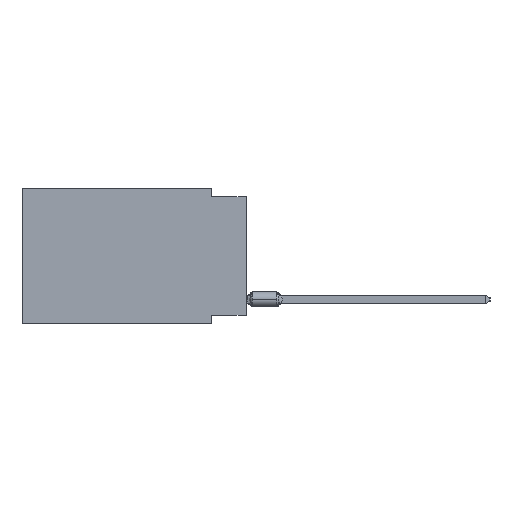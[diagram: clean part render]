
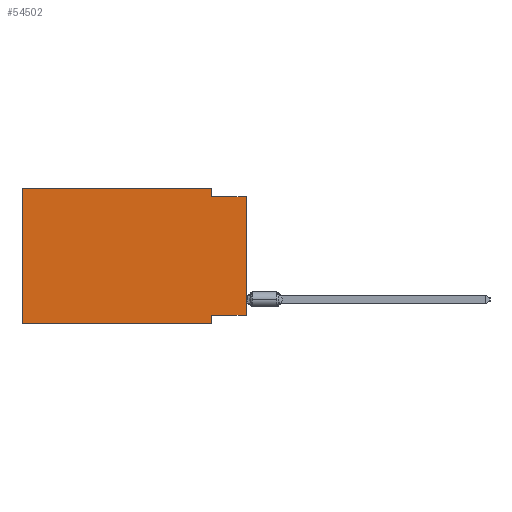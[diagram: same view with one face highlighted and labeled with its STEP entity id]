
A CAD part, left-side view. The second image highlights one B-rep face of the part: STEP entity #54502.
In plain terms, the highlighted planar face has unit normal (-1, 0, 0).
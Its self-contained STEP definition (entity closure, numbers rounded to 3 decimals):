
#494 = EDGE_LOOP ( 'NONE', ( #45677, #50648, #28081, #15392, #49542, #27873, #43400, #24106 ) ) ;
#1900 = DIRECTION ( 'NONE',  ( 0., -1., 0. ) ) ;
#3722 = VERTEX_POINT ( 'NONE', #21673 ) ;
#4236 = DIRECTION ( 'NONE',  ( 0., 0., 1. ) ) ;
#6100 = DIRECTION ( 'NONE',  ( 0., 0., -1. ) ) ;
#8981 = CARTESIAN_POINT ( 'NONE',  ( 0., 16.383, 0. ) ) ;
#9177 = DIRECTION ( 'NONE',  ( 1., 0., 0. ) ) ;
#10129 = VERTEX_POINT ( 'NONE', #53542 ) ;
#11128 = VECTOR ( 'NONE', #14428, 1000. ) ;
#11525 = LINE ( 'NONE', #20707, #32580 ) ;
#12353 = CARTESIAN_POINT ( 'NONE',  ( 0., 2.54, 0. ) ) ;
#14428 = DIRECTION ( 'NONE',  ( 0., 0., 1. ) ) ;
#15392 = ORIENTED_EDGE ( 'NONE', *, *, #49906, .F. ) ;
#15967 = DIRECTION ( 'NONE',  ( 0., 0., -1. ) ) ;
#17964 = VERTEX_POINT ( 'NONE', #32989 ) ;
#18384 = FACE_OUTER_BOUND ( 'NONE', #494, .T. ) ;
#19208 = LINE ( 'NONE', #40193, #21951 ) ;
#20163 = DIRECTION ( 'NONE',  ( 0., -1., 0. ) ) ;
#20707 = CARTESIAN_POINT ( 'NONE',  ( 0., 16.383, 0. ) ) ;
#20918 = AXIS2_PLACEMENT_3D ( 'NONE', #22013, #9177, #6100 ) ;
#21673 = CARTESIAN_POINT ( 'NONE',  ( 0., 16.383, 0. ) ) ;
#21951 = VECTOR ( 'NONE', #1900, 1000. ) ;
#22013 = CARTESIAN_POINT ( 'NONE',  ( 0., 16.383, 0. ) ) ;
#22137 = EDGE_CURVE ( 'NONE', #49790, #39181, #42387, .T. ) ;
#23502 = CARTESIAN_POINT ( 'NONE',  ( 0., 2.54, -9.906 ) ) ;
#24106 = ORIENTED_EDGE ( 'NONE', *, *, #32005, .F. ) ;
#25196 = LINE ( 'NONE', #29409, #46056 ) ;
#25326 = DIRECTION ( 'NONE',  ( 0., 0., -1. ) ) ;
#26961 = EDGE_CURVE ( 'NONE', #32284, #39181, #19208, .T. ) ;
#27005 = EDGE_CURVE ( 'NONE', #32284, #3722, #38580, .T. ) ;
#27210 = VERTEX_POINT ( 'NONE', #52263 ) ;
#27873 = ORIENTED_EDGE ( 'NONE', *, *, #26961, .T. ) ;
#28081 = ORIENTED_EDGE ( 'NONE', *, *, #48700, .F. ) ;
#28136 = VECTOR ( 'NONE', #15967, 1000. ) ;
#29409 = CARTESIAN_POINT ( 'NONE',  ( 0., 0., -0.635 ) ) ;
#30150 = VERTEX_POINT ( 'NONE', #50470 ) ;
#30831 = CARTESIAN_POINT ( 'NONE',  ( 0., 2.54, -9.906 ) ) ;
#32005 = EDGE_CURVE ( 'NONE', #30150, #49790, #45163, .T. ) ;
#32284 = VERTEX_POINT ( 'NONE', #44002 ) ;
#32580 = VECTOR ( 'NONE', #20163, 1000. ) ;
#32845 = VECTOR ( 'NONE', #25326, 1000. ) ;
#32989 = CARTESIAN_POINT ( 'NONE',  ( 0., 2.54, 0. ) ) ;
#35422 = LINE ( 'NONE', #52452, #11128 ) ;
#38282 = VECTOR ( 'NONE', #54097, 1000. ) ;
#38580 = LINE ( 'NONE', #8981, #53182 ) ;
#39181 = VERTEX_POINT ( 'NONE', #23502 ) ;
#40193 = CARTESIAN_POINT ( 'NONE',  ( 0., 16.383, -9.906 ) ) ;
#42387 = LINE ( 'NONE', #30831, #32845 ) ;
#43400 = ORIENTED_EDGE ( 'NONE', *, *, #22137, .F. ) ;
#44002 = CARTESIAN_POINT ( 'NONE',  ( 0., 16.383, -9.906 ) ) ;
#44405 = EDGE_CURVE ( 'NONE', #30150, #10129, #35422, .T. ) ;
#45163 = LINE ( 'NONE', #45990, #38282 ) ;
#45677 = ORIENTED_EDGE ( 'NONE', *, *, #44405, .T. ) ;
#45930 = EDGE_CURVE ( 'NONE', #27210, #10129, #25196, .T. ) ;
#45990 = CARTESIAN_POINT ( 'NONE',  ( 0., 0., -9.271 ) ) ;
#46056 = VECTOR ( 'NONE', #46449, 1000. ) ;
#46449 = DIRECTION ( 'NONE',  ( 0., -1., 0. ) ) ;
#48700 = EDGE_CURVE ( 'NONE', #17964, #27210, #54542, .T. ) ;
#49542 = ORIENTED_EDGE ( 'NONE', *, *, #27005, .F. ) ;
#49790 = VERTEX_POINT ( 'NONE', #52614 ) ;
#49906 = EDGE_CURVE ( 'NONE', #3722, #17964, #11525, .T. ) ;
#50470 = CARTESIAN_POINT ( 'NONE',  ( 0., 0., -9.271 ) ) ;
#50648 = ORIENTED_EDGE ( 'NONE', *, *, #45930, .F. ) ;
#52263 = CARTESIAN_POINT ( 'NONE',  ( 0., 2.54, -0.635 ) ) ;
#52452 = CARTESIAN_POINT ( 'NONE',  ( 0., 0., 0. ) ) ;
#52476 = PLANE ( 'NONE',  #20918 ) ;
#52614 = CARTESIAN_POINT ( 'NONE',  ( 0., 2.54, -9.271 ) ) ;
#53182 = VECTOR ( 'NONE', #4236, 1000. ) ;
#53542 = CARTESIAN_POINT ( 'NONE',  ( 0., 0., -0.635 ) ) ;
#54097 = DIRECTION ( 'NONE',  ( 0., 1., 0. ) ) ;
#54502 = ADVANCED_FACE ( 'NONE', ( #18384 ), #52476, .F. ) ;
#54542 = LINE ( 'NONE', #12353, #28136 ) ;
